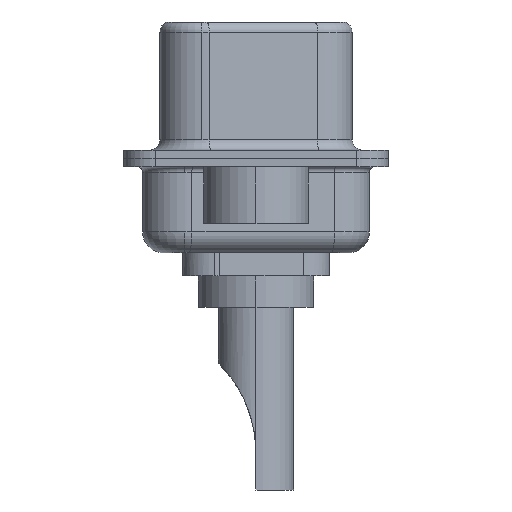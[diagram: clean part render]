
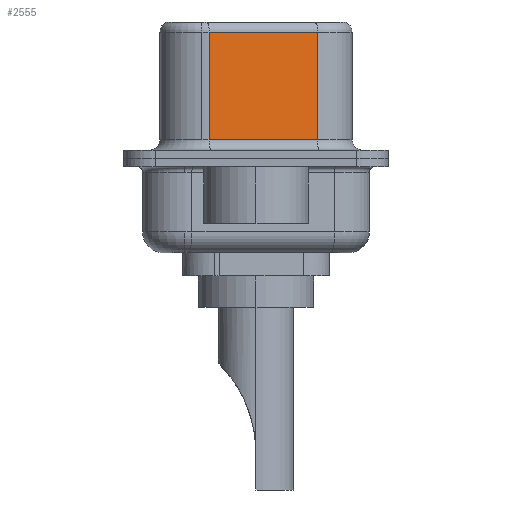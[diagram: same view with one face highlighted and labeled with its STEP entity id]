
A CAD part, left-side view. The second image highlights one B-rep face of the part: STEP entity #2555.
In plain terms, the highlighted planar face has unit normal (-0.985, -0.174, 0).
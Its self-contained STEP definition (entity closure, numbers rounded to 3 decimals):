
#517 = EDGE_CURVE ( 'NONE', #8339, #10288, #4146, .T. ) ;
#671 = ORIENTED_EDGE ( 'NONE', *, *, #4528, .T. ) ;
#1214 = CARTESIAN_POINT ( 'NONE',  ( 3.675, 2.233, 6.02 ) ) ;
#1293 = VERTEX_POINT ( 'NONE', #7974 ) ;
#1441 = VECTOR ( 'NONE', #13898, 1000. ) ;
#1874 = PLANE ( 'NONE',  #5697 ) ;
#2072 = VECTOR ( 'NONE', #13264, 1000. ) ;
#2234 = EDGE_LOOP ( 'NONE', ( #14277, #13207, #12508, #671 ) ) ;
#2555 = ADVANCED_FACE ( 'NONE', ( #9594 ), #1874, .F. ) ;
#3274 = EDGE_CURVE ( 'NONE', #1293, #8339, #11144, .T. ) ;
#4029 = LINE ( 'NONE', #12531, #12613 ) ;
#4146 = LINE ( 'NONE', #8820, #1441 ) ;
#4528 = EDGE_CURVE ( 'NONE', #10288, #9467, #9549, .T. ) ;
#4674 = EDGE_CURVE ( 'NONE', #1293, #9467, #4029, .T. ) ;
#4700 = DIRECTION ( 'NONE',  ( 0.174, -0.985, 0. ) ) ;
#5661 = CARTESIAN_POINT ( 'NONE',  ( 4.585, -2.927, 6.52 ) ) ;
#5697 = AXIS2_PLACEMENT_3D ( 'NONE', #5661, #7052, #11943 ) ;
#5699 = CARTESIAN_POINT ( 'NONE',  ( 3.675, 2.233, 0.9 ) ) ;
#6603 = VECTOR ( 'NONE', #4700, 1000. ) ;
#6942 = DIRECTION ( 'NONE',  ( 0., 0., -1. ) ) ;
#7052 = DIRECTION ( 'NONE',  ( 0.985, 0.174, 0. ) ) ;
#7974 = CARTESIAN_POINT ( 'NONE',  ( 4.585, -2.927, 6.02 ) ) ;
#8339 = VERTEX_POINT ( 'NONE', #1214 ) ;
#8820 = CARTESIAN_POINT ( 'NONE',  ( 3.675, 2.233, 6.52 ) ) ;
#9467 = VERTEX_POINT ( 'NONE', #13804 ) ;
#9549 = LINE ( 'NONE', #14322, #6603 ) ;
#9594 = FACE_OUTER_BOUND ( 'NONE', #2234, .T. ) ;
#10288 = VERTEX_POINT ( 'NONE', #5699 ) ;
#11144 = LINE ( 'NONE', #13246, #2072 ) ;
#11943 = DIRECTION ( 'NONE',  ( -0.174, 0.985, 0. ) ) ;
#12508 = ORIENTED_EDGE ( 'NONE', *, *, #517, .T. ) ;
#12531 = CARTESIAN_POINT ( 'NONE',  ( 4.585, -2.927, 6.52 ) ) ;
#12613 = VECTOR ( 'NONE', #6942, 1000. ) ;
#13207 = ORIENTED_EDGE ( 'NONE', *, *, #3274, .T. ) ;
#13246 = CARTESIAN_POINT ( 'NONE',  ( 4.585, -2.927, 6.02 ) ) ;
#13264 = DIRECTION ( 'NONE',  ( -0.174, 0.985, 0. ) ) ;
#13804 = CARTESIAN_POINT ( 'NONE',  ( 4.585, -2.927, 0.9 ) ) ;
#13898 = DIRECTION ( 'NONE',  ( 0., 0., -1. ) ) ;
#14277 = ORIENTED_EDGE ( 'NONE', *, *, #4674, .F. ) ;
#14322 = CARTESIAN_POINT ( 'NONE',  ( 4.585, -2.927, 0.9 ) ) ;
